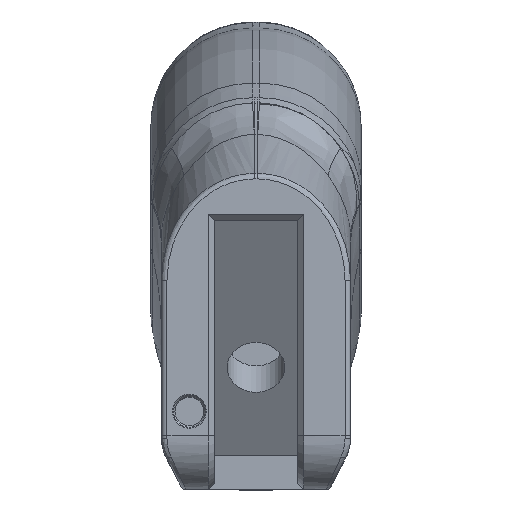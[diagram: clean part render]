
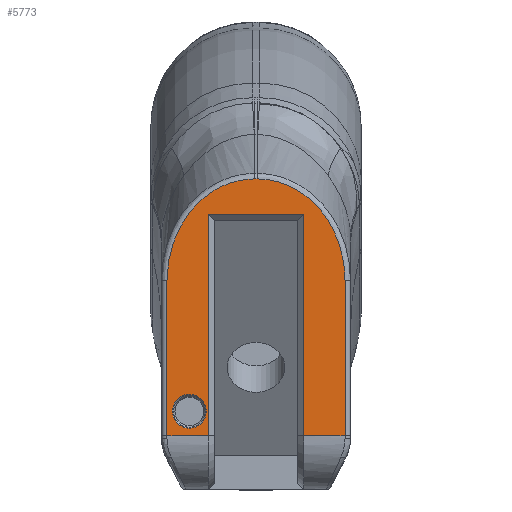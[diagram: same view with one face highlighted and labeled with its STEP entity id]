
A CAD part, top view. The second image highlights one B-rep face of the part: STEP entity #5773.
In plain terms, the highlighted planar face has unit normal (0, 0, 1).
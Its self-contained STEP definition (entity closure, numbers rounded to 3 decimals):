
#80=LINE('',#13064,#235);
#82=LINE('',#13078,#237);
#84=LINE('',#13133,#239);
#111=LINE('',#14280,#266);
#112=LINE('',#14384,#267);
#116=LINE('',#14393,#271);
#125=LINE('',#14444,#280);
#126=LINE('',#14445,#281);
#235=VECTOR('',#6956,10.);
#237=VECTOR('',#6966,10.);
#239=VECTOR('',#6982,10.);
#266=VECTOR('',#7227,10.);
#267=VECTOR('',#7232,10.);
#271=VECTOR('',#7240,10.);
#280=VECTOR('',#7261,10.);
#281=VECTOR('',#7262,10.);
#380=FACE_BOUND('',#1126,.T.);
#414=PLANE('',#6292);
#737=FACE_OUTER_BOUND('',#1125,.T.);
#1125=EDGE_LOOP('',(#4638,#4639,#4640,#4641,#4642,#4643,#4644,#4645,#4646,
#4647));
#1126=EDGE_LOOP('',(#4648));
#1483=B_SPLINE_CURVE_WITH_KNOTS('',3,(#13196,#13197,#13198,#13199,#13200,
#13201,#13202,#13203,#13204,#13205,#13206,#13207),.UNSPECIFIED.,.F.,.F.,
(4,2,2,2,2,4),(0.,0.598,0.939,1.3,
1.578,1.752),.UNSPECIFIED.);
#1530=B_SPLINE_CURVE_WITH_KNOTS('',3,(#14344,#14345,#14346,#14347,#14348,
#14349,#14350,#14351,#14352,#14353,#14354,#14355),.UNSPECIFIED.,.F.,.F.,
(4,2,2,2,2,4),(0.,0.174,0.453,0.814,
1.155,1.75),.UNSPECIFIED.);
#1760=CIRCLE('',#6044,2.);
#2108=VERTEX_POINT('',#9344);
#2304=VERTEX_POINT('',#13058);
#2305=VERTEX_POINT('',#13062);
#2307=VERTEX_POINT('',#13068);
#2310=VERTEX_POINT('',#13132);
#2311=VERTEX_POINT('',#13195);
#2407=VERTEX_POINT('',#14274);
#2408=VERTEX_POINT('',#14278);
#2410=VERTEX_POINT('',#14342);
#2415=VERTEX_POINT('',#14383);
#2416=VERTEX_POINT('',#14387);
#2707=EDGE_CURVE('',#2108,#2108,#1760,.T.);
#3020=EDGE_CURVE('',#2305,#2304,#80,.T.);
#3025=EDGE_CURVE('',#2307,#2304,#82,.T.);
#3031=EDGE_CURVE('',#2307,#2310,#84,.T.);
#3033=EDGE_CURVE('',#2310,#2311,#1483,.T.);
#3180=EDGE_CURVE('',#2408,#2407,#111,.T.);
#3182=EDGE_CURVE('',#2410,#2408,#1530,.T.);
#3188=EDGE_CURVE('',#2407,#2415,#112,.T.);
#3193=EDGE_CURVE('',#2415,#2416,#116,.T.);
#3203=EDGE_CURVE('',#2416,#2305,#125,.T.);
#3204=EDGE_CURVE('',#2311,#2410,#126,.T.);
#4638=ORIENTED_EDGE('',*,*,#3203,.F.);
#4639=ORIENTED_EDGE('',*,*,#3193,.F.);
#4640=ORIENTED_EDGE('',*,*,#3188,.F.);
#4641=ORIENTED_EDGE('',*,*,#3180,.F.);
#4642=ORIENTED_EDGE('',*,*,#3182,.F.);
#4643=ORIENTED_EDGE('',*,*,#3204,.F.);
#4644=ORIENTED_EDGE('',*,*,#3033,.F.);
#4645=ORIENTED_EDGE('',*,*,#3031,.F.);
#4646=ORIENTED_EDGE('',*,*,#3025,.T.);
#4647=ORIENTED_EDGE('',*,*,#3020,.F.);
#4648=ORIENTED_EDGE('',*,*,#2707,.F.);
#5773=ADVANCED_FACE('',(#737,#380),#414,.T.);
#6044=AXIS2_PLACEMENT_3D('',#9345,#6666,#6667);
#6292=AXIS2_PLACEMENT_3D('',#14443,#7259,#7260);
#6666=DIRECTION('center_axis',(0.,0.,
1.));
#6667=DIRECTION('ref_axis',(1.,0.,0.));
#6956=DIRECTION('',(0.,-1.,0.));
#6966=DIRECTION('',(1.,0.,0.));
#6982=DIRECTION('',(0.,1.,0.));
#7227=DIRECTION('',(0.,-1.,0.));
#7232=DIRECTION('',(-1.,0.,0.));
#7240=DIRECTION('',(0.,1.,0.));
#7259=DIRECTION('center_axis',(0.,0.,
1.));
#7260=DIRECTION('ref_axis',(0.,-1.,0.));
#7261=DIRECTION('',(-1.,0.,0.));
#7262=DIRECTION('',(1.,0.,0.));
#9344=CARTESIAN_POINT('',(14.205,-140.572,28.406));
#9345=CARTESIAN_POINT('Origin',(16.205,-140.572,28.406));
#13058=CARTESIAN_POINT('',(18.417,-143.468,28.406));
#13062=CARTESIAN_POINT('',(18.417,-117.318,28.406));
#13064=CARTESIAN_POINT('',(18.417,-114.618,28.406));
#13068=CARTESIAN_POINT('',(13.568,-143.468,28.406));
#13078=CARTESIAN_POINT('',(28.956,-143.468,28.406));
#13132=CARTESIAN_POINT('',(13.568,-125.147,28.406));
#13133=CARTESIAN_POINT('',(13.568,-40.367,28.406));
#13195=CARTESIAN_POINT('',(23.918,-113.127,28.406));
#13196=CARTESIAN_POINT('Ctrl Pts',(13.568,-125.147,28.406));
#13197=CARTESIAN_POINT('Ctrl Pts',(13.568,-123.155,28.406));
#13198=CARTESIAN_POINT('Ctrl Pts',(13.998,-121.15,28.406));
#13199=CARTESIAN_POINT('Ctrl Pts',(15.342,-118.318,28.406));
#13200=CARTESIAN_POINT('Ctrl Pts',(15.978,-117.342,28.406));
#13201=CARTESIAN_POINT('Ctrl Pts',(17.546,-115.588,28.406));
#13202=CARTESIAN_POINT('Ctrl Pts',(18.499,-114.817,28.406));
#13203=CARTESIAN_POINT('Ctrl Pts',(20.387,-113.8,28.406));
#13204=CARTESIAN_POINT('Ctrl Pts',(21.265,-113.479,28.406));
#13205=CARTESIAN_POINT('Ctrl Pts',(22.756,-113.184,28.406));
#13206=CARTESIAN_POINT('Ctrl Pts',(23.339,-113.127,28.406));
#13207=CARTESIAN_POINT('Ctrl Pts',(23.918,-113.127,28.406));
#14274=CARTESIAN_POINT('',(34.595,-143.468,28.406));
#14278=CARTESIAN_POINT('',(34.595,-125.147,28.406));
#14280=CARTESIAN_POINT('',(34.595,-40.367,28.406));
#14342=CARTESIAN_POINT('',(24.245,-113.127,28.406));
#14344=CARTESIAN_POINT('Ctrl Pts',(24.245,-113.127,28.406));
#14345=CARTESIAN_POINT('Ctrl Pts',(24.826,-113.127,28.406));
#14346=CARTESIAN_POINT('Ctrl Pts',(25.41,-113.184,28.406));
#14347=CARTESIAN_POINT('Ctrl Pts',(26.893,-113.478,28.406));
#14348=CARTESIAN_POINT('Ctrl Pts',(27.775,-113.799,28.406));
#14349=CARTESIAN_POINT('Ctrl Pts',(29.662,-114.815,28.406));
#14350=CARTESIAN_POINT('Ctrl Pts',(30.618,-115.589,28.406));
#14351=CARTESIAN_POINT('Ctrl Pts',(32.182,-117.337,28.406));
#14352=CARTESIAN_POINT('Ctrl Pts',(32.819,-118.315,28.406));
#14353=CARTESIAN_POINT('Ctrl Pts',(34.163,-121.144,28.406));
#14354=CARTESIAN_POINT('Ctrl Pts',(34.595,-123.163,28.406));
#14355=CARTESIAN_POINT('Ctrl Pts',(34.595,-125.147,28.406));
#14383=CARTESIAN_POINT('',(29.746,-143.468,28.406));
#14384=CARTESIAN_POINT('',(19.207,-143.468,28.406));
#14387=CARTESIAN_POINT('',(29.746,-117.318,28.406));
#14393=CARTESIAN_POINT('',(29.746,-114.618,28.406));
#14443=CARTESIAN_POINT('Origin',(19.207,-112.624,28.406));
#14444=CARTESIAN_POINT('',(24.173,-117.318,28.406));
#14445=CARTESIAN_POINT('',(27.226,-113.127,28.406));
